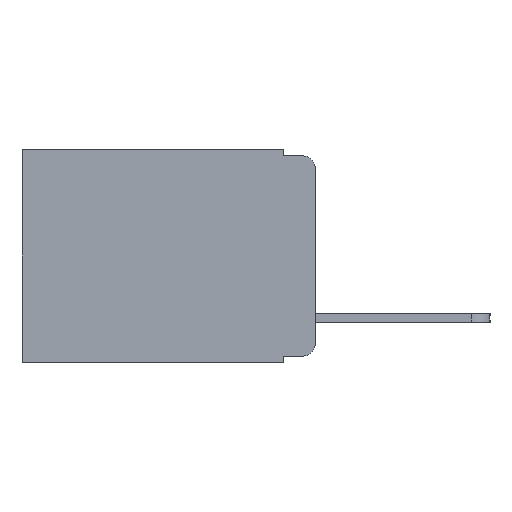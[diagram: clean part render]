
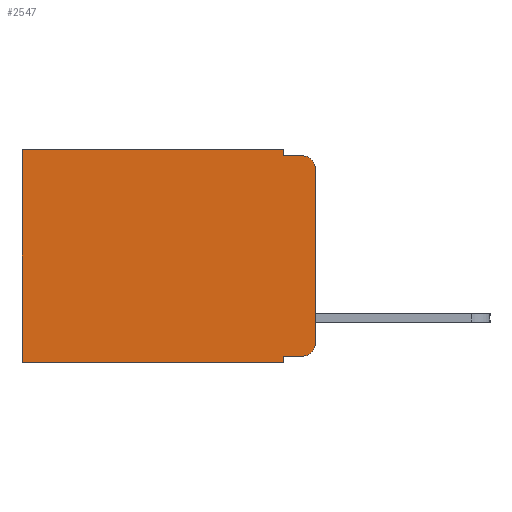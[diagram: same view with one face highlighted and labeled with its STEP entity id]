
A CAD part, left-side view. The second image highlights one B-rep face of the part: STEP entity #2547.
In plain terms, the highlighted planar face has unit normal (-1, 0, 0).
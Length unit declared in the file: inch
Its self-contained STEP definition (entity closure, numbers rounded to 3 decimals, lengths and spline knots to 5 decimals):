
#124 = LINE ( 'NONE', #9520, #5580 ) ;
#290 = EDGE_CURVE ( 'NONE', #6095, #11009, #124, .T. ) ;
#367 = CARTESIAN_POINT ( 'NONE',  ( 0.298, 0.473, 0. ) ) ;
#386 = VERTEX_POINT ( 'NONE', #678 ) ;
#438 = CARTESIAN_POINT ( 'NONE',  ( 0.298, 0., -0.313 ) ) ;
#678 = CARTESIAN_POINT ( 'NONE',  ( 0.298, 0., -0.03 ) ) ;
#938 = EDGE_LOOP ( 'NONE', ( #4438, #4328, #4684, #4540, #4770, #12547, #9055, #5337, #9636, #7604 ) ) ;
#1035 = VECTOR ( 'NONE', #5911, 39.37008 ) ;
#1109 = VERTEX_POINT ( 'NONE', #4654 ) ;
#1544 = DIRECTION ( 'NONE',  ( 0., 0., -1. ) ) ;
#1606 = CARTESIAN_POINT ( 'NONE',  ( 0.298, 0.02, -0.313 ) ) ;
#1626 = DIRECTION ( 'NONE',  ( -1., 0., 0. ) ) ;
#2030 = CARTESIAN_POINT ( 'NONE',  ( 0.298, 0.02, -0.03 ) ) ;
#2547 = ADVANCED_FACE ( 'NONE', ( #3537 ), #12500, .F. ) ;
#2765 = VERTEX_POINT ( 'NONE', #438 ) ;
#2919 = LINE ( 'NONE', #7612, #7977 ) ;
#2952 = CARTESIAN_POINT ( 'NONE',  ( 0.298, 0.02, -0.333 ) ) ;
#2996 = CIRCLE ( 'NONE', #5738, 0.02 ) ;
#3149 = DIRECTION ( 'NONE',  ( 0., 0., -1. ) ) ;
#3381 = DIRECTION ( 'NONE',  ( 0., 1., 0. ) ) ;
#3389 = VECTOR ( 'NONE', #10469, 39.37008 ) ;
#3537 = FACE_OUTER_BOUND ( 'NONE', #938, .T. ) ;
#3761 = EDGE_CURVE ( 'NONE', #12652, #2765, #2996, .T. ) ;
#3972 = CARTESIAN_POINT ( 'NONE',  ( 0.298, 0.051, 0. ) ) ;
#4065 = VECTOR ( 'NONE', #6902, 39.37008 ) ;
#4328 = ORIENTED_EDGE ( 'NONE', *, *, #10721, .T. ) ;
#4438 = ORIENTED_EDGE ( 'NONE', *, *, #6820, .F. ) ;
#4540 = ORIENTED_EDGE ( 'NONE', *, *, #10576, .F. ) ;
#4654 = CARTESIAN_POINT ( 'NONE',  ( 0.298, 0.051, -0.333 ) ) ;
#4684 = ORIENTED_EDGE ( 'NONE', *, *, #290, .F. ) ;
#4704 = AXIS2_PLACEMENT_3D ( 'NONE', #2030, #9126, #3149 ) ;
#4770 = ORIENTED_EDGE ( 'NONE', *, *, #8668, .T. ) ;
#4843 = VERTEX_POINT ( 'NONE', #11150 ) ;
#4879 = VERTEX_POINT ( 'NONE', #9924 ) ;
#5203 = VERTEX_POINT ( 'NONE', #11345 ) ;
#5337 = ORIENTED_EDGE ( 'NONE', *, *, #11949, .F. ) ;
#5554 = CARTESIAN_POINT ( 'NONE',  ( 0.298, 0.02, -0.01 ) ) ;
#5580 = VECTOR ( 'NONE', #8812, 39.37008 ) ;
#5621 = LINE ( 'NONE', #6676, #12548 ) ;
#5738 = AXIS2_PLACEMENT_3D ( 'NONE', #1606, #1626, #1544 ) ;
#5911 = DIRECTION ( 'NONE',  ( 0., 0., -1. ) ) ;
#6061 = VECTOR ( 'NONE', #9839, 39.37008 ) ;
#6095 = VERTEX_POINT ( 'NONE', #8949 ) ;
#6536 = AXIS2_PLACEMENT_3D ( 'NONE', #12570, #11621, #11490 ) ;
#6598 = VECTOR ( 'NONE', #7539, 39.37008 ) ;
#6632 = LINE ( 'NONE', #3972, #6061 ) ;
#6676 = CARTESIAN_POINT ( 'NONE',  ( 0.298, 0., 0. ) ) ;
#6727 = LINE ( 'NONE', #7861, #4065 ) ;
#6740 = LINE ( 'NONE', #9941, #3389 ) ;
#6820 = EDGE_CURVE ( 'NONE', #386, #2765, #6740, .T. ) ;
#6874 = LINE ( 'NONE', #8517, #6598 ) ;
#6902 = DIRECTION ( 'NONE',  ( 0., 1., 0. ) ) ;
#7053 = CIRCLE ( 'NONE', #4704, 0.02 ) ;
#7408 = VERTEX_POINT ( 'NONE', #10260 ) ;
#7539 = DIRECTION ( 'NONE',  ( 0., 0., -1. ) ) ;
#7604 = ORIENTED_EDGE ( 'NONE', *, *, #3761, .T. ) ;
#7612 = CARTESIAN_POINT ( 'NONE',  ( 0.298, 0.051, -0.333 ) ) ;
#7861 = CARTESIAN_POINT ( 'NONE',  ( 0.298, 0., -0.343 ) ) ;
#7977 = VECTOR ( 'NONE', #9534, 39.37008 ) ;
#8517 = CARTESIAN_POINT ( 'NONE',  ( 0.298, 0.051, 0. ) ) ;
#8668 = EDGE_CURVE ( 'NONE', #4879, #4843, #5621, .T. ) ;
#8812 = DIRECTION ( 'NONE',  ( 0., -1., 0. ) ) ;
#8949 = CARTESIAN_POINT ( 'NONE',  ( 0.298, 0.051, -0.01 ) ) ;
#9055 = ORIENTED_EDGE ( 'NONE', *, *, #12197, .F. ) ;
#9126 = DIRECTION ( 'NONE',  ( -1., 0., 0. ) ) ;
#9520 = CARTESIAN_POINT ( 'NONE',  ( 0.298, 0.051, -0.01 ) ) ;
#9534 = DIRECTION ( 'NONE',  ( 0., -1., 0. ) ) ;
#9598 = LINE ( 'NONE', #367, #1035 ) ;
#9636 = ORIENTED_EDGE ( 'NONE', *, *, #11139, .T. ) ;
#9839 = DIRECTION ( 'NONE',  ( 0., 0., -1. ) ) ;
#9924 = CARTESIAN_POINT ( 'NONE',  ( 0.298, 0.051, 0. ) ) ;
#9941 = CARTESIAN_POINT ( 'NONE',  ( 0.298, 0., 0. ) ) ;
#10260 = CARTESIAN_POINT ( 'NONE',  ( 0.298, 0.051, -0.343 ) ) ;
#10469 = DIRECTION ( 'NONE',  ( 0., 0., -1. ) ) ;
#10576 = EDGE_CURVE ( 'NONE', #4879, #6095, #6632, .T. ) ;
#10721 = EDGE_CURVE ( 'NONE', #386, #11009, #7053, .T. ) ;
#11009 = VERTEX_POINT ( 'NONE', #5554 ) ;
#11139 = EDGE_CURVE ( 'NONE', #1109, #12652, #2919, .T. ) ;
#11150 = CARTESIAN_POINT ( 'NONE',  ( 0.298, 0.473, 0. ) ) ;
#11291 = EDGE_CURVE ( 'NONE', #4843, #5203, #9598, .T. ) ;
#11345 = CARTESIAN_POINT ( 'NONE',  ( 0.298, 0.473, -0.343 ) ) ;
#11490 = DIRECTION ( 'NONE',  ( 0., 0., -1. ) ) ;
#11621 = DIRECTION ( 'NONE',  ( 1., 0., 0. ) ) ;
#11949 = EDGE_CURVE ( 'NONE', #1109, #7408, #6874, .T. ) ;
#12197 = EDGE_CURVE ( 'NONE', #7408, #5203, #6727, .T. ) ;
#12500 = PLANE ( 'NONE',  #6536 ) ;
#12547 = ORIENTED_EDGE ( 'NONE', *, *, #11291, .T. ) ;
#12548 = VECTOR ( 'NONE', #3381, 39.37008 ) ;
#12570 = CARTESIAN_POINT ( 'NONE',  ( 0.298, 0., 0. ) ) ;
#12652 = VERTEX_POINT ( 'NONE', #2952 ) ;
